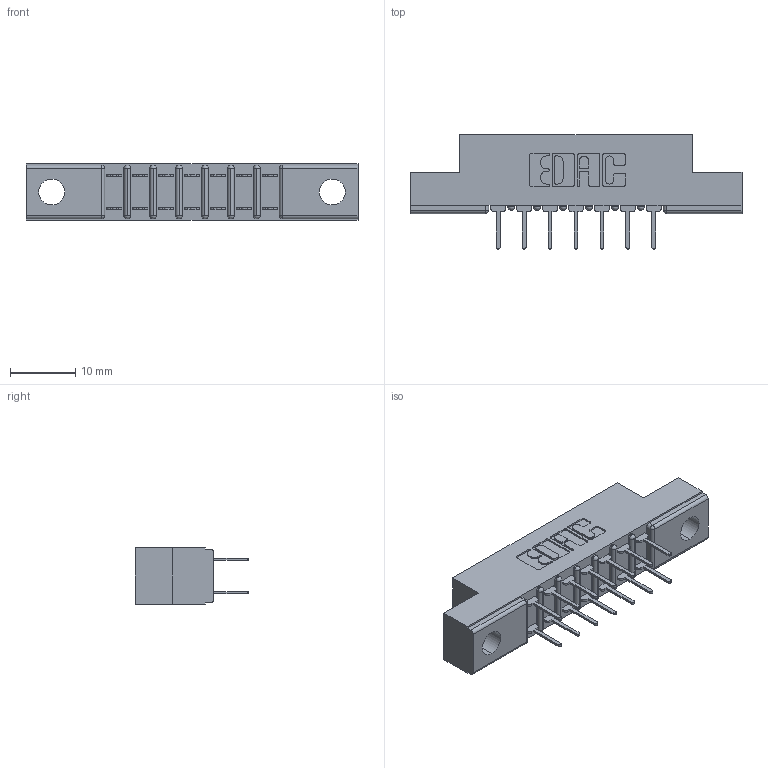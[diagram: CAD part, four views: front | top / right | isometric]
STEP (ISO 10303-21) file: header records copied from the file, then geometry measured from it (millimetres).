
FILE_DESCRIPTION (( 'STEP AP203' ), '1' );
FILE_NAME ('307-014-424-204.STEP', '2020-09-28T15:45:01', ( '' ), ( '' ), 'SwSTEP 2.0', 'SolidWorks 2020', '' );
FILE_SCHEMA (( 'CONFIG_CONTROL_DESIGN' ));
Length unit declared in the file: inch
Products named in the file (9): 307-014-424-204; 307 Part_.156 Dia Mounting Holes; 307-290-001_524; 345-250-001_345-250-005-103; 307-014-424-207; #22580; #35014
Assembly tree (77 placements, depth 2):
  307-014-424-204
    307 Part_.156 Dia Mounting Holes
    307-290-001_524  x14
  307-014-424-207
    307 Part_.156 Dia Mounting Holes
    307-290-001_524  x14
    345-250-001_345-250-005-103  x2
  #35014
    #22580
    #17330  x42
    #20547  x2
Bounding box: 50.75 x 17.42 x 8.71 mm (x, y, z)
Volume: 3210.7 mm3; surface area: 4753.3 mm2
Topology: 15 solids, 15 shells, 784 faces, 2179 edges, 1410 vertices
Faces by surface type: plane 518, cylinder 250, sphere 16
Entity records: 37474 total; most frequent: CARTESIAN_POINT 6145, ORIENTED_EDGE 6141, DIRECTION 6064, EDGE_CURVE 3065, LINE 2362, VECTOR 2307, VERTEX_POINT 1988, AXIS2_PLACEMENT_3D 1891
